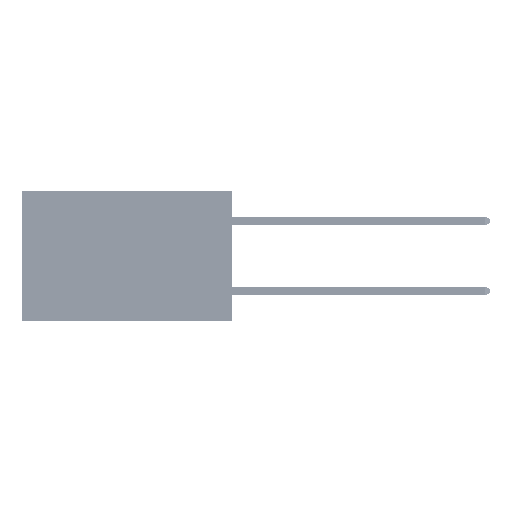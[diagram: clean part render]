
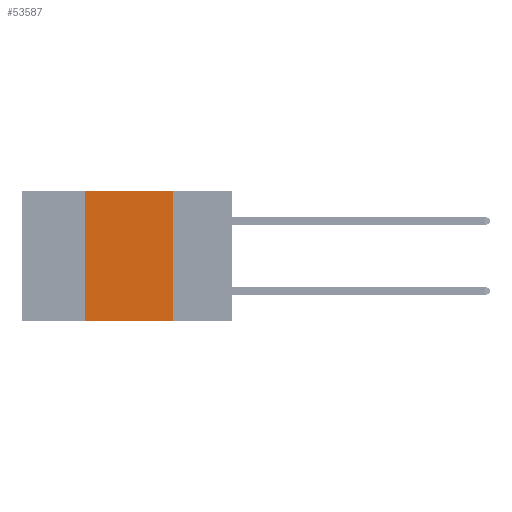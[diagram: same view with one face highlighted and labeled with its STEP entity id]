
A CAD part, left-side view. The second image highlights one B-rep face of the part: STEP entity #53587.
In plain terms, the highlighted planar face has unit normal (-1, 0, 0).
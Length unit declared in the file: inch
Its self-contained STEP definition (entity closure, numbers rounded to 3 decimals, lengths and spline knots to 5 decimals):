
#643 = EDGE_LOOP ( 'NONE', ( #38198, #11099, #11807, #16774 ) ) ;
#1060 = VERTEX_POINT ( 'NONE', #41363 ) ;
#2355 = VECTOR ( 'NONE', #19417, 39.37008 ) ;
#4354 = FACE_OUTER_BOUND ( 'NONE', #643, .T. ) ;
#5248 = VECTOR ( 'NONE', #15782, 39.37008 ) ;
#5884 = AXIS2_PLACEMENT_3D ( 'NONE', #16074, #37544, #12665 ) ;
#7098 = VECTOR ( 'NONE', #30815, 39.37008 ) ;
#7887 = LINE ( 'NONE', #19769, #5248 ) ;
#8379 = CARTESIAN_POINT ( 'NONE',  ( 0., 0.42, 0. ) ) ;
#10479 = VERTEX_POINT ( 'NONE', #38220 ) ;
#11019 = LINE ( 'NONE', #11695, #50009 ) ;
#11099 = ORIENTED_EDGE ( 'NONE', *, *, #39506, .F. ) ;
#11137 = CARTESIAN_POINT ( 'NONE',  ( 0., 0.6, -0.37 ) ) ;
#11695 = CARTESIAN_POINT ( 'NONE',  ( 0., 0.17, 0. ) ) ;
#11807 = ORIENTED_EDGE ( 'NONE', *, *, #27482, .F. ) ;
#12665 = DIRECTION ( 'NONE',  ( 0., 0., -1. ) ) ;
#12732 = LINE ( 'NONE', #11137, #2355 ) ;
#15782 = DIRECTION ( 'NONE',  ( 0., -1., 0. ) ) ;
#16074 = CARTESIAN_POINT ( 'NONE',  ( 0., 0.6, 0. ) ) ;
#16774 = ORIENTED_EDGE ( 'NONE', *, *, #33191, .T. ) ;
#19417 = DIRECTION ( 'NONE',  ( 0., -1., 0. ) ) ;
#19769 = CARTESIAN_POINT ( 'NONE',  ( 0., 0.6, 0. ) ) ;
#24650 = PLANE ( 'NONE',  #5884 ) ;
#27482 = EDGE_CURVE ( 'NONE', #28960, #46515, #29189, .T. ) ;
#28960 = VERTEX_POINT ( 'NONE', #41465 ) ;
#29189 = LINE ( 'NONE', #8379, #7098 ) ;
#30672 = EDGE_CURVE ( 'NONE', #10479, #1060, #11019, .T. ) ;
#30815 = DIRECTION ( 'NONE',  ( 0., 0., 1. ) ) ;
#33191 = EDGE_CURVE ( 'NONE', #28960, #1060, #12732, .T. ) ;
#37544 = DIRECTION ( 'NONE',  ( 1., 0., 0. ) ) ;
#38198 = ORIENTED_EDGE ( 'NONE', *, *, #30672, .F. ) ;
#38220 = CARTESIAN_POINT ( 'NONE',  ( 0., 0.17, 0. ) ) ;
#39506 = EDGE_CURVE ( 'NONE', #46515, #10479, #7887, .T. ) ;
#41363 = CARTESIAN_POINT ( 'NONE',  ( 0., 0.17, -0.37 ) ) ;
#41465 = CARTESIAN_POINT ( 'NONE',  ( 0., 0.42, -0.37 ) ) ;
#46515 = VERTEX_POINT ( 'NONE', #52859 ) ;
#50009 = VECTOR ( 'NONE', #53438, 39.37008 ) ;
#52859 = CARTESIAN_POINT ( 'NONE',  ( 0., 0.42, 0. ) ) ;
#53438 = DIRECTION ( 'NONE',  ( 0., 0., -1. ) ) ;
#53587 = ADVANCED_FACE ( 'NONE', ( #4354 ), #24650, .F. ) ;
